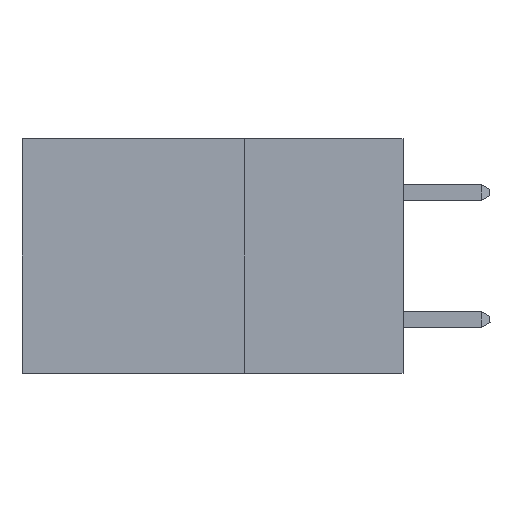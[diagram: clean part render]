
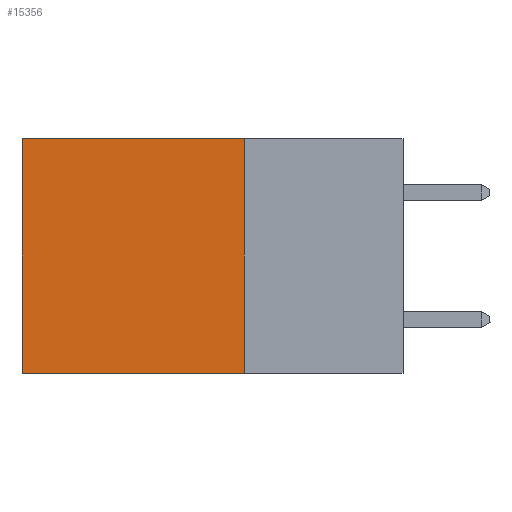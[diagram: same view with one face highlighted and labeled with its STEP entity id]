
A CAD part, left-side view. The second image highlights one B-rep face of the part: STEP entity #15356.
In plain terms, the highlighted planar face has unit normal (-1, 0, 0).
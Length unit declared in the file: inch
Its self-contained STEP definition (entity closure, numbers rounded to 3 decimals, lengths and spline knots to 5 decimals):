
#4082 = EDGE_CURVE ( 'NONE', #18723, #6236, #7977, .T. ) ;
#5211 = EDGE_CURVE ( 'NONE', #6236, #27508, #21635, .T. ) ;
#5232 = DIRECTION ( 'NONE',  ( 0., 0., -1. ) ) ;
#5258 = VERTEX_POINT ( 'NONE', #25698 ) ;
#6236 = VERTEX_POINT ( 'NONE', #22595 ) ;
#6320 = CARTESIAN_POINT ( 'NONE',  ( 0.2875, 0.25, 0. ) ) ;
#6485 = DIRECTION ( 'NONE',  ( 1., 0., 0. ) ) ;
#6594 = ORIENTED_EDGE ( 'NONE', *, *, #7234, .F. ) ;
#6828 = VECTOR ( 'NONE', #22968, 39.37008 ) ;
#7234 = EDGE_CURVE ( 'NONE', #18723, #5258, #8211, .T. ) ;
#7340 = FACE_OUTER_BOUND ( 'NONE', #11144, .T. ) ;
#7752 = DIRECTION ( 'NONE',  ( 0., 1., 0. ) ) ;
#7977 = LINE ( 'NONE', #9571, #25178 ) ;
#8211 = LINE ( 'NONE', #6320, #19670 ) ;
#9099 = PLANE ( 'NONE',  #16456 ) ;
#9571 = CARTESIAN_POINT ( 'NONE',  ( 0.2875, 0.25, 0. ) ) ;
#9615 = ORIENTED_EDGE ( 'NONE', *, *, #11487, .F. ) ;
#10323 = CARTESIAN_POINT ( 'NONE',  ( 0.2875, 0.6, 0. ) ) ;
#10869 = VECTOR ( 'NONE', #5232, 39.37008 ) ;
#11135 = CARTESIAN_POINT ( 'NONE',  ( 0.2875, 0.25, 0. ) ) ;
#11144 = EDGE_LOOP ( 'NONE', ( #14483, #9615, #6594, #20938 ) ) ;
#11487 = EDGE_CURVE ( 'NONE', #5258, #27508, #12952, .T. ) ;
#11517 = DIRECTION ( 'NONE',  ( 0., 0., -1. ) ) ;
#12952 = LINE ( 'NONE', #18553, #6828 ) ;
#14483 = ORIENTED_EDGE ( 'NONE', *, *, #5211, .T. ) ;
#15356 = ADVANCED_FACE ( 'NONE', ( #7340 ), #9099, .F. ) ;
#15910 = DIRECTION ( 'NONE',  ( 0., 0., -1. ) ) ;
#16456 = AXIS2_PLACEMENT_3D ( 'NONE', #22526, #6485, #11517 ) ;
#18553 = CARTESIAN_POINT ( 'NONE',  ( 0.2875, 0.25, -0.37 ) ) ;
#18723 = VERTEX_POINT ( 'NONE', #11135 ) ;
#19670 = VECTOR ( 'NONE', #15910, 39.37008 ) ;
#19689 = CARTESIAN_POINT ( 'NONE',  ( 0.2875, 0.6, -0.37 ) ) ;
#20938 = ORIENTED_EDGE ( 'NONE', *, *, #4082, .T. ) ;
#21635 = LINE ( 'NONE', #10323, #10869 ) ;
#22526 = CARTESIAN_POINT ( 'NONE',  ( 0.2875, 0.25, 0. ) ) ;
#22595 = CARTESIAN_POINT ( 'NONE',  ( 0.2875, 0.6, 0. ) ) ;
#22968 = DIRECTION ( 'NONE',  ( 0., 1., 0. ) ) ;
#25178 = VECTOR ( 'NONE', #7752, 39.37008 ) ;
#25698 = CARTESIAN_POINT ( 'NONE',  ( 0.2875, 0.25, -0.37 ) ) ;
#27508 = VERTEX_POINT ( 'NONE', #19689 ) ;
